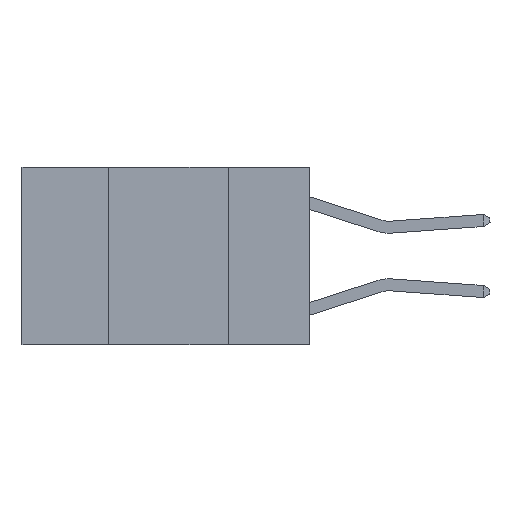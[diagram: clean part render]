
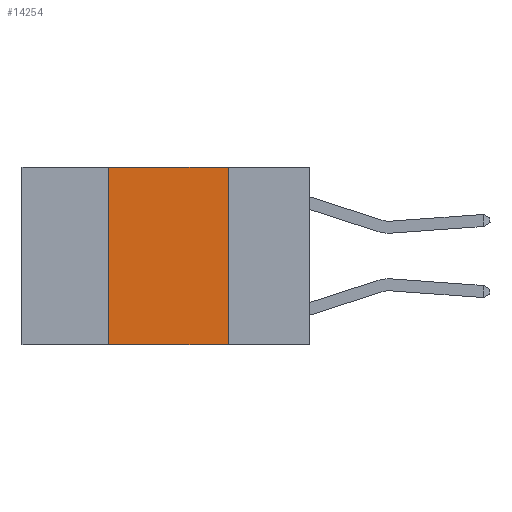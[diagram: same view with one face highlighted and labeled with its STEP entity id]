
A CAD part, left-side view. The second image highlights one B-rep face of the part: STEP entity #14254.
In plain terms, the highlighted planar face has unit normal (-1, 0, 0).
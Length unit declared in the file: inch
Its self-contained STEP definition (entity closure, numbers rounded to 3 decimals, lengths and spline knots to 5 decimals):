
#1175 = VECTOR ( 'NONE', #23160, 39.37008 ) ;
#1792 = CARTESIAN_POINT ( 'NONE',  ( 0., 0.17, -0.37 ) ) ;
#2344 = PLANE ( 'NONE',  #7229 ) ;
#3623 = CARTESIAN_POINT ( 'NONE',  ( 0., 0.42, 0. ) ) ;
#3877 = ORIENTED_EDGE ( 'NONE', *, *, #8805, .F. ) ;
#4193 = LINE ( 'NONE', #8518, #26601 ) ;
#5230 = VERTEX_POINT ( 'NONE', #3623 ) ;
#5862 = DIRECTION ( 'NONE',  ( 0., 0., -1. ) ) ;
#6659 = FACE_OUTER_BOUND ( 'NONE', #24993, .T. ) ;
#7229 = AXIS2_PLACEMENT_3D ( 'NONE', #26341, #11413, #13367 ) ;
#8518 = CARTESIAN_POINT ( 'NONE',  ( 0., 0.6, 0. ) ) ;
#8623 = CARTESIAN_POINT ( 'NONE',  ( 0., 0.42, 0. ) ) ;
#8805 = EDGE_CURVE ( 'NONE', #14721, #27488, #27228, .T. ) ;
#10949 = ORIENTED_EDGE ( 'NONE', *, *, #24063, .T. ) ;
#11413 = DIRECTION ( 'NONE',  ( 1., 0., 0. ) ) ;
#13367 = DIRECTION ( 'NONE',  ( 0., 0., -1. ) ) ;
#14005 = CARTESIAN_POINT ( 'NONE',  ( 0., 0.42, -0.37 ) ) ;
#14254 = ADVANCED_FACE ( 'NONE', ( #6659 ), #2344, .F. ) ;
#14303 = ORIENTED_EDGE ( 'NONE', *, *, #21634, .F. ) ;
#14721 = VERTEX_POINT ( 'NONE', #19348 ) ;
#15982 = VECTOR ( 'NONE', #5862, 39.37008 ) ;
#17660 = CARTESIAN_POINT ( 'NONE',  ( 0., 0.6, -0.37 ) ) ;
#18871 = CARTESIAN_POINT ( 'NONE',  ( 0., 0.17, 0. ) ) ;
#19245 = LINE ( 'NONE', #8623, #1175 ) ;
#19347 = DIRECTION ( 'NONE',  ( 0., -1., 0. ) ) ;
#19348 = CARTESIAN_POINT ( 'NONE',  ( 0., 0.17, 0. ) ) ;
#20820 = VECTOR ( 'NONE', #19347, 39.37008 ) ;
#21589 = ORIENTED_EDGE ( 'NONE', *, *, #23463, .F. ) ;
#21634 = EDGE_CURVE ( 'NONE', #5230, #14721, #4193, .T. ) ;
#21861 = LINE ( 'NONE', #17660, #20820 ) ;
#23160 = DIRECTION ( 'NONE',  ( 0., 0., 1. ) ) ;
#23463 = EDGE_CURVE ( 'NONE', #24334, #5230, #19245, .T. ) ;
#24063 = EDGE_CURVE ( 'NONE', #24334, #27488, #21861, .T. ) ;
#24334 = VERTEX_POINT ( 'NONE', #14005 ) ;
#24993 = EDGE_LOOP ( 'NONE', ( #3877, #14303, #21589, #10949 ) ) ;
#26341 = CARTESIAN_POINT ( 'NONE',  ( 0., 0.6, 0. ) ) ;
#26601 = VECTOR ( 'NONE', #27216, 39.37008 ) ;
#27216 = DIRECTION ( 'NONE',  ( 0., -1., 0. ) ) ;
#27228 = LINE ( 'NONE', #18871, #15982 ) ;
#27488 = VERTEX_POINT ( 'NONE', #1792 ) ;
